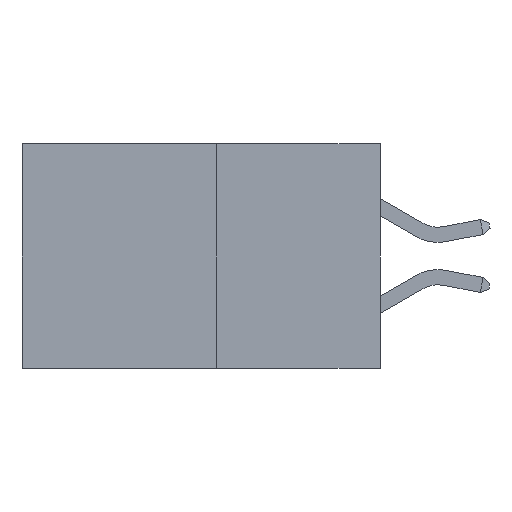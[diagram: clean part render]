
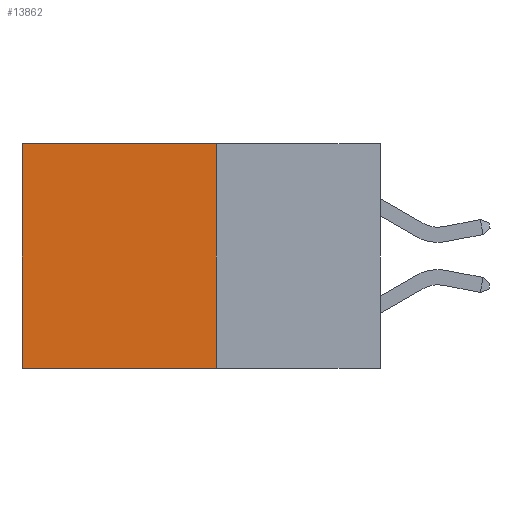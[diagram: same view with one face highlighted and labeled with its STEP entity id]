
A CAD part, left-side view. The second image highlights one B-rep face of the part: STEP entity #13862.
In plain terms, the highlighted planar face has unit normal (-1, 0, 0).
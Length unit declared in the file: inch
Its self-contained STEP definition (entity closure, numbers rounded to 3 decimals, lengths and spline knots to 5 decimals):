
#1911 = VECTOR ( 'NONE', #2947, 39.37008 ) ;
#2067 = CARTESIAN_POINT ( 'NONE',  ( 0.277, 0.59, -0.37 ) ) ;
#2383 = CARTESIAN_POINT ( 'NONE',  ( 0.277, 0.27, -0.37 ) ) ;
#2947 = DIRECTION ( 'NONE',  ( 0., 1., 0. ) ) ;
#3677 = CARTESIAN_POINT ( 'NONE',  ( 0.277, 0.27, 0. ) ) ;
#5335 = EDGE_CURVE ( 'NONE', #5385, #11217, #24798, .T. ) ;
#5385 = VERTEX_POINT ( 'NONE', #20354 ) ;
#6706 = VECTOR ( 'NONE', #27779, 39.37008 ) ;
#6776 = DIRECTION ( 'NONE',  ( 0., 0., -1. ) ) ;
#7568 = CARTESIAN_POINT ( 'NONE',  ( 0.277, 0.27, -0.37 ) ) ;
#9452 = CARTESIAN_POINT ( 'NONE',  ( 0.277, 0.59, -0.37 ) ) ;
#9574 = LINE ( 'NONE', #2067, #25867 ) ;
#10808 = CARTESIAN_POINT ( 'NONE',  ( 0.277, 0.27, -0.37 ) ) ;
#11217 = VERTEX_POINT ( 'NONE', #16039 ) ;
#11449 = EDGE_LOOP ( 'NONE', ( #18984, #12578, #26432, #20059 ) ) ;
#11706 = FACE_OUTER_BOUND ( 'NONE', #11449, .T. ) ;
#12578 = ORIENTED_EDGE ( 'NONE', *, *, #24777, .F. ) ;
#13862 = ADVANCED_FACE ( 'NONE', ( #11706 ), #15393, .F. ) ;
#13996 = EDGE_CURVE ( 'NONE', #5385, #23511, #18749, .T. ) ;
#15393 = PLANE ( 'NONE',  #19270 ) ;
#16039 = CARTESIAN_POINT ( 'NONE',  ( 0.277, 0.59, 0. ) ) ;
#17542 = EDGE_CURVE ( 'NONE', #11217, #25845, #9574, .T. ) ;
#18749 = LINE ( 'NONE', #7568, #23790 ) ;
#18984 = ORIENTED_EDGE ( 'NONE', *, *, #17542, .T. ) ;
#19270 = AXIS2_PLACEMENT_3D ( 'NONE', #2383, #19658, #6776 ) ;
#19339 = DIRECTION ( 'NONE',  ( 0., 0., -1. ) ) ;
#19658 = DIRECTION ( 'NONE',  ( 1., 0., 0. ) ) ;
#20059 = ORIENTED_EDGE ( 'NONE', *, *, #5335, .T. ) ;
#20354 = CARTESIAN_POINT ( 'NONE',  ( 0.277, 0.27, 0. ) ) ;
#21443 = CARTESIAN_POINT ( 'NONE',  ( 0.277, 0.27, -0.37 ) ) ;
#23511 = VERTEX_POINT ( 'NONE', #21443 ) ;
#23790 = VECTOR ( 'NONE', #24670, 39.37008 ) ;
#24480 = LINE ( 'NONE', #10808, #6706 ) ;
#24670 = DIRECTION ( 'NONE',  ( 0., 0., -1. ) ) ;
#24777 = EDGE_CURVE ( 'NONE', #23511, #25845, #24480, .T. ) ;
#24798 = LINE ( 'NONE', #3677, #1911 ) ;
#25845 = VERTEX_POINT ( 'NONE', #9452 ) ;
#25867 = VECTOR ( 'NONE', #19339, 39.37008 ) ;
#26432 = ORIENTED_EDGE ( 'NONE', *, *, #13996, .F. ) ;
#27779 = DIRECTION ( 'NONE',  ( 0., 1., 0. ) ) ;
